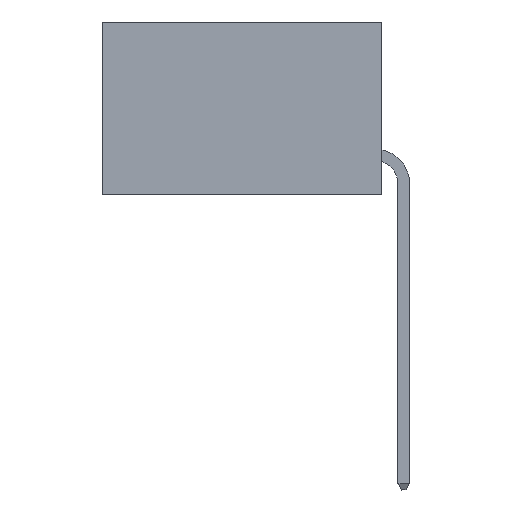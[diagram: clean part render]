
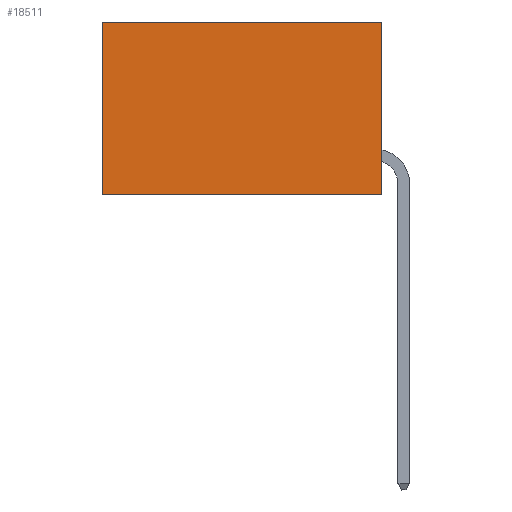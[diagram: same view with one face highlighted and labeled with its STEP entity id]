
A CAD part, left-side view. The second image highlights one B-rep face of the part: STEP entity #18511.
In plain terms, the highlighted planar face has unit normal (-1, 0, 0).
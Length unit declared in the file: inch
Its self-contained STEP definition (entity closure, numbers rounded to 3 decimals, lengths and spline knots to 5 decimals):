
#357 = LINE ( 'NONE', #17780, #10936 ) ;
#1133 = CARTESIAN_POINT ( 'NONE',  ( 0.2875, 0., 0. ) ) ;
#1527 = CARTESIAN_POINT ( 'NONE',  ( 0.2875, 0., 0. ) ) ;
#1811 = DIRECTION ( 'NONE',  ( 0., 1., 0. ) ) ;
#2358 = ORIENTED_EDGE ( 'NONE', *, *, #17461, .T. ) ;
#5407 = VERTEX_POINT ( 'NONE', #25572 ) ;
#5564 = FACE_OUTER_BOUND ( 'NONE', #9764, .T. ) ;
#6829 = EDGE_CURVE ( 'NONE', #5407, #12452, #34268, .T. ) ;
#7155 = ORIENTED_EDGE ( 'NONE', *, *, #17350, .F. ) ;
#7202 = CARTESIAN_POINT ( 'NONE',  ( 0.2875, 0.6, 0. ) ) ;
#8843 = VERTEX_POINT ( 'NONE', #32974 ) ;
#9149 = VECTOR ( 'NONE', #16182, 39.37008 ) ;
#9278 = EDGE_CURVE ( 'NONE', #8843, #32784, #34624, .T. ) ;
#9472 = CARTESIAN_POINT ( 'NONE',  ( 0.2875, 0., -0.37 ) ) ;
#9764 = EDGE_LOOP ( 'NONE', ( #16132, #7155, #22200, #2358 ) ) ;
#10936 = VECTOR ( 'NONE', #1811, 39.37008 ) ;
#11103 = PLANE ( 'NONE',  #31847 ) ;
#12452 = VERTEX_POINT ( 'NONE', #12951 ) ;
#12951 = CARTESIAN_POINT ( 'NONE',  ( 0.2875, 0.6, -0.37 ) ) ;
#13729 = DIRECTION ( 'NONE',  ( 1., 0., 0. ) ) ;
#16132 = ORIENTED_EDGE ( 'NONE', *, *, #6829, .T. ) ;
#16182 = DIRECTION ( 'NONE',  ( 0., 1., 0. ) ) ;
#16254 = VECTOR ( 'NONE', #34758, 39.37008 ) ;
#17350 = EDGE_CURVE ( 'NONE', #32784, #12452, #357, .T. ) ;
#17461 = EDGE_CURVE ( 'NONE', #8843, #5407, #21938, .T. ) ;
#17780 = CARTESIAN_POINT ( 'NONE',  ( 0.2875, 0., -0.37 ) ) ;
#18511 = ADVANCED_FACE ( 'NONE', ( #5564 ), #11103, .F. ) ;
#19589 = DIRECTION ( 'NONE',  ( 0., 0., -1. ) ) ;
#21938 = LINE ( 'NONE', #1527, #9149 ) ;
#22200 = ORIENTED_EDGE ( 'NONE', *, *, #9278, .F. ) ;
#24866 = CARTESIAN_POINT ( 'NONE',  ( 0.2875, 0., 0. ) ) ;
#25572 = CARTESIAN_POINT ( 'NONE',  ( 0.2875, 0.6, 0. ) ) ;
#31847 = AXIS2_PLACEMENT_3D ( 'NONE', #24866, #13729, #19589 ) ;
#32108 = VECTOR ( 'NONE', #34803, 39.37008 ) ;
#32784 = VERTEX_POINT ( 'NONE', #9472 ) ;
#32974 = CARTESIAN_POINT ( 'NONE',  ( 0.2875, 0., 0. ) ) ;
#34268 = LINE ( 'NONE', #7202, #32108 ) ;
#34624 = LINE ( 'NONE', #1133, #16254 ) ;
#34758 = DIRECTION ( 'NONE',  ( 0., 0., -1. ) ) ;
#34803 = DIRECTION ( 'NONE',  ( 0., 0., -1. ) ) ;
